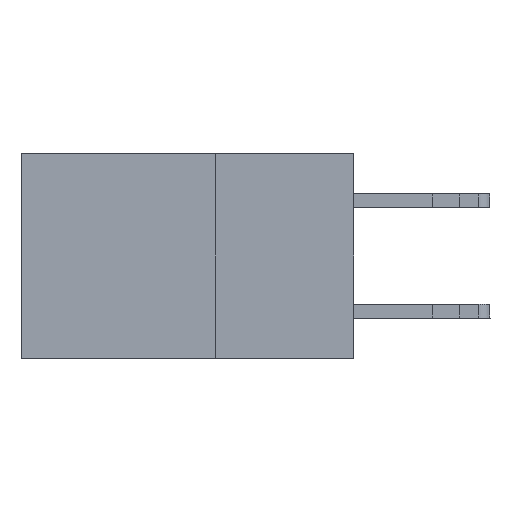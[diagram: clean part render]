
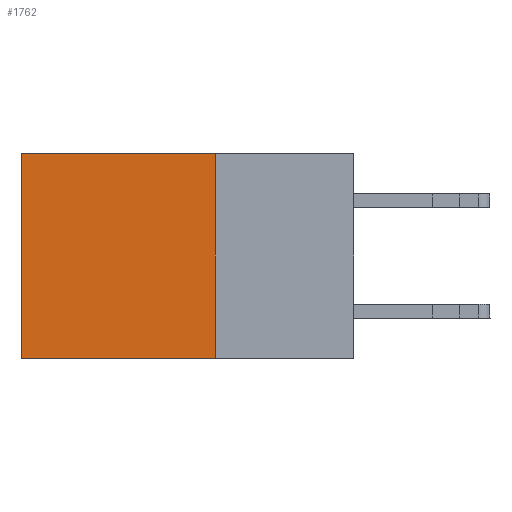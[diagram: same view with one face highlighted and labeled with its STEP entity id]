
A CAD part, left-side view. The second image highlights one B-rep face of the part: STEP entity #1762.
In plain terms, the highlighted planar face has unit normal (-1, 0, 0).
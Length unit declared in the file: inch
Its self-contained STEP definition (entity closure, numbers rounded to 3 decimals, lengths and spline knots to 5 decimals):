
#928 = VECTOR ( 'NONE', #12356, 39.37008 ) ;
#934 = EDGE_CURVE ( 'NONE', #22156, #7021, #8416, .T. ) ;
#1082 = ORIENTED_EDGE ( 'NONE', *, *, #5404, .F. ) ;
#1142 = CARTESIAN_POINT ( 'NONE',  ( 0.2875, 0.25, -0.37 ) ) ;
#1236 = AXIS2_PLACEMENT_3D ( 'NONE', #2824, #23252, #6527 ) ;
#1762 = ADVANCED_FACE ( 'NONE', ( #16590 ), #25515, .F. ) ;
#2824 = CARTESIAN_POINT ( 'NONE',  ( 0.2875, 0.25, 0. ) ) ;
#4837 = EDGE_LOOP ( 'NONE', ( #13839, #1082, #23932, #15335 ) ) ;
#5404 = EDGE_CURVE ( 'NONE', #7021, #10457, #11852, .T. ) ;
#6266 = VECTOR ( 'NONE', #17065, 39.37008 ) ;
#6527 = DIRECTION ( 'NONE',  ( 0., 0., -1. ) ) ;
#7021 = VERTEX_POINT ( 'NONE', #1142 ) ;
#7335 = CARTESIAN_POINT ( 'NONE',  ( 0.2875, 0.25, 0. ) ) ;
#8416 = LINE ( 'NONE', #22492, #18892 ) ;
#9256 = VERTEX_POINT ( 'NONE', #14247 ) ;
#10292 = EDGE_CURVE ( 'NONE', #9256, #10457, #19124, .T. ) ;
#10457 = VERTEX_POINT ( 'NONE', #25522 ) ;
#11852 = LINE ( 'NONE', #20305, #6266 ) ;
#12356 = DIRECTION ( 'NONE',  ( 0., 1., 0. ) ) ;
#13839 = ORIENTED_EDGE ( 'NONE', *, *, #10292, .T. ) ;
#14247 = CARTESIAN_POINT ( 'NONE',  ( 0.2875, 0.6, 0. ) ) ;
#15335 = ORIENTED_EDGE ( 'NONE', *, *, #20549, .T. ) ;
#16590 = FACE_OUTER_BOUND ( 'NONE', #4837, .T. ) ;
#16623 = LINE ( 'NONE', #18857, #928 ) ;
#17065 = DIRECTION ( 'NONE',  ( 0., 1., 0. ) ) ;
#17996 = CARTESIAN_POINT ( 'NONE',  ( 0.2875, 0.6, 0. ) ) ;
#18857 = CARTESIAN_POINT ( 'NONE',  ( 0.2875, 0.25, 0. ) ) ;
#18892 = VECTOR ( 'NONE', #20140, 39.37008 ) ;
#19124 = LINE ( 'NONE', #17996, #23350 ) ;
#20140 = DIRECTION ( 'NONE',  ( 0., 0., -1. ) ) ;
#20305 = CARTESIAN_POINT ( 'NONE',  ( 0.2875, 0.25, -0.37 ) ) ;
#20549 = EDGE_CURVE ( 'NONE', #22156, #9256, #16623, .T. ) ;
#22156 = VERTEX_POINT ( 'NONE', #7335 ) ;
#22492 = CARTESIAN_POINT ( 'NONE',  ( 0.2875, 0.25, 0. ) ) ;
#22544 = DIRECTION ( 'NONE',  ( 0., 0., -1. ) ) ;
#23252 = DIRECTION ( 'NONE',  ( 1., 0., 0. ) ) ;
#23350 = VECTOR ( 'NONE', #22544, 39.37008 ) ;
#23932 = ORIENTED_EDGE ( 'NONE', *, *, #934, .F. ) ;
#25515 = PLANE ( 'NONE',  #1236 ) ;
#25522 = CARTESIAN_POINT ( 'NONE',  ( 0.2875, 0.6, -0.37 ) ) ;
